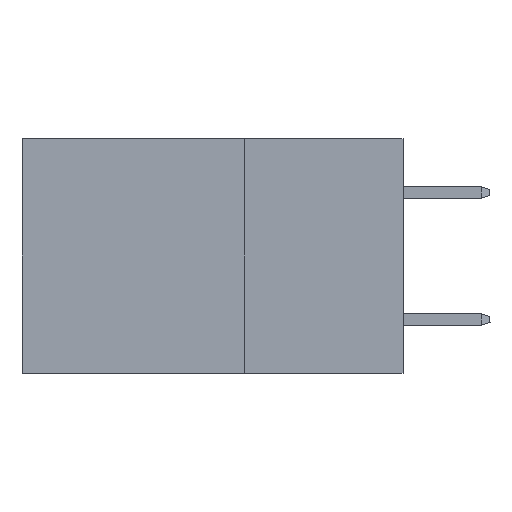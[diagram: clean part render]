
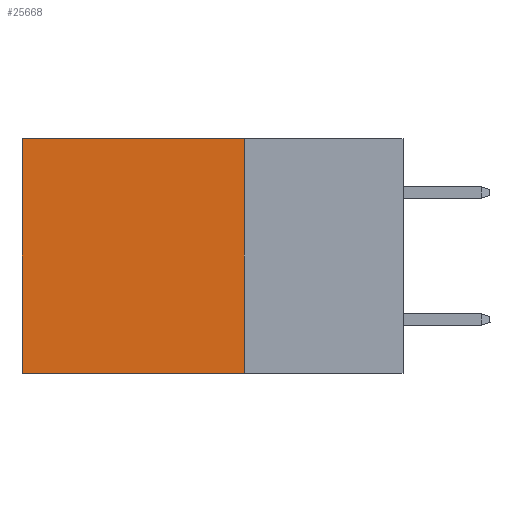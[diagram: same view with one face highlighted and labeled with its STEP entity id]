
A CAD part, left-side view. The second image highlights one B-rep face of the part: STEP entity #25668.
In plain terms, the highlighted planar face has unit normal (-1, 0, 0).
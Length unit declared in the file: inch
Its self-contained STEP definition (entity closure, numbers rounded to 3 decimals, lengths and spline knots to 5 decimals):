
#46 = CARTESIAN_POINT ( 'NONE',  ( 0.2875, 0.25, -0.37 ) ) ;
#1634 = DIRECTION ( 'NONE',  ( 1., 0., 0. ) ) ;
#3246 = VERTEX_POINT ( 'NONE', #20068 ) ;
#3639 = VERTEX_POINT ( 'NONE', #24058 ) ;
#4225 = LINE ( 'NONE', #22156, #4652 ) ;
#4405 = ORIENTED_EDGE ( 'NONE', *, *, #13718, .T. ) ;
#4652 = VECTOR ( 'NONE', #22418, 39.37008 ) ;
#5632 = CARTESIAN_POINT ( 'NONE',  ( 0.2875, 0.25, 0. ) ) ;
#6200 = EDGE_CURVE ( 'NONE', #24039, #19338, #14972, .T. ) ;
#7058 = ORIENTED_EDGE ( 'NONE', *, *, #6200, .T. ) ;
#8238 = DIRECTION ( 'NONE',  ( 0., 0., -1. ) ) ;
#8976 = VECTOR ( 'NONE', #17099, 39.37008 ) ;
#9768 = EDGE_LOOP ( 'NONE', ( #4405, #15792, #24821, #7058 ) ) ;
#11495 = VECTOR ( 'NONE', #8238, 39.37008 ) ;
#12231 = DIRECTION ( 'NONE',  ( 0., 0., -1. ) ) ;
#12404 = CARTESIAN_POINT ( 'NONE',  ( 0.2875, 0.25, 0. ) ) ;
#13718 = EDGE_CURVE ( 'NONE', #19338, #3639, #4225, .T. ) ;
#14114 = EDGE_CURVE ( 'NONE', #24039, #3246, #14265, .T. ) ;
#14265 = LINE ( 'NONE', #12404, #11495 ) ;
#14315 = VECTOR ( 'NONE', #24789, 39.37008 ) ;
#14714 = CARTESIAN_POINT ( 'NONE',  ( 0.2875, 0.25, 0. ) ) ;
#14741 = AXIS2_PLACEMENT_3D ( 'NONE', #5632, #1634, #12231 ) ;
#14972 = LINE ( 'NONE', #14714, #8976 ) ;
#15792 = ORIENTED_EDGE ( 'NONE', *, *, #21357, .F. ) ;
#16118 = LINE ( 'NONE', #46, #14315 ) ;
#16359 = FACE_OUTER_BOUND ( 'NONE', #9768, .T. ) ;
#16780 = CARTESIAN_POINT ( 'NONE',  ( 0.2875, 0.25, 0. ) ) ;
#17099 = DIRECTION ( 'NONE',  ( 0., 1., 0. ) ) ;
#19338 = VERTEX_POINT ( 'NONE', #25379 ) ;
#19845 = PLANE ( 'NONE',  #14741 ) ;
#20068 = CARTESIAN_POINT ( 'NONE',  ( 0.2875, 0.25, -0.37 ) ) ;
#21357 = EDGE_CURVE ( 'NONE', #3246, #3639, #16118, .T. ) ;
#22156 = CARTESIAN_POINT ( 'NONE',  ( 0.2875, 0.6, 0. ) ) ;
#22418 = DIRECTION ( 'NONE',  ( 0., 0., -1. ) ) ;
#24039 = VERTEX_POINT ( 'NONE', #16780 ) ;
#24058 = CARTESIAN_POINT ( 'NONE',  ( 0.2875, 0.6, -0.37 ) ) ;
#24789 = DIRECTION ( 'NONE',  ( 0., 1., 0. ) ) ;
#24821 = ORIENTED_EDGE ( 'NONE', *, *, #14114, .F. ) ;
#25379 = CARTESIAN_POINT ( 'NONE',  ( 0.2875, 0.6, 0. ) ) ;
#25668 = ADVANCED_FACE ( 'NONE', ( #16359 ), #19845, .F. ) ;
